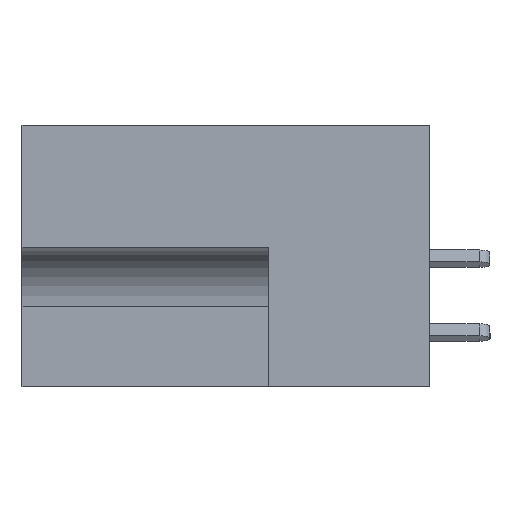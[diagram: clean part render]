
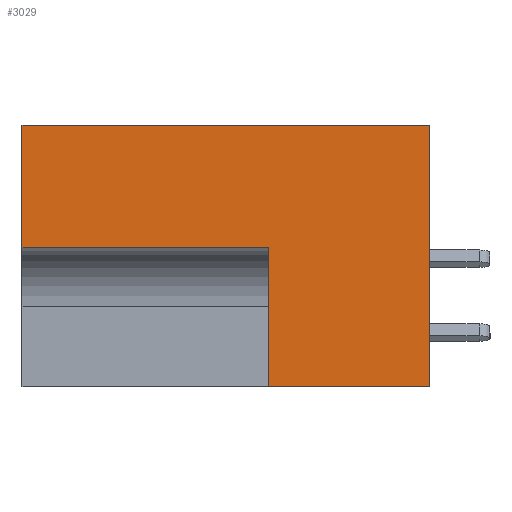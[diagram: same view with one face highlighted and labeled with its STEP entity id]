
A CAD part, left-side view. The second image highlights one B-rep face of the part: STEP entity #3029.
In plain terms, the highlighted planar face has unit normal (-1, 0, 0).
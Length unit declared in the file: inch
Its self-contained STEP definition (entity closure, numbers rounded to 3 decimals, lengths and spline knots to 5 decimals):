
#59 = EDGE_CURVE ( 'NONE', #28640, #12085, #19210, .T. ) ;
#116 = CARTESIAN_POINT ( 'NONE',  ( 0., 0.828, 0. ) ) ;
#3029 = ADVANCED_FACE ( 'NONE', ( #16331 ), #13114, .F. ) ;
#4414 = ORIENTED_EDGE ( 'NONE', *, *, #17054, .T. ) ;
#4541 = CARTESIAN_POINT ( 'NONE',  ( 0., 0.328, -0.248 ) ) ;
#5088 = CARTESIAN_POINT ( 'NONE',  ( 0., 0., -0.531 ) ) ;
#5208 = EDGE_CURVE ( 'NONE', #25098, #28640, #22709, .T. ) ;
#5227 = VECTOR ( 'NONE', #7574, 39.37008 ) ;
#5331 = VECTOR ( 'NONE', #13494, 39.37008 ) ;
#5976 = CARTESIAN_POINT ( 'NONE',  ( 0., 0.328, -0.248 ) ) ;
#7574 = DIRECTION ( 'NONE',  ( 0., 0., 1. ) ) ;
#8869 = EDGE_CURVE ( 'NONE', #22255, #29161, #20364, .T. ) ;
#9506 = LINE ( 'NONE', #26531, #28365 ) ;
#9760 = DIRECTION ( 'NONE',  ( 0., -1., 0. ) ) ;
#10424 = ORIENTED_EDGE ( 'NONE', *, *, #8869, .F. ) ;
#10444 = CARTESIAN_POINT ( 'NONE',  ( 0., 0.328, -0.531 ) ) ;
#12024 = CARTESIAN_POINT ( 'NONE',  ( 0., 0.453, 0. ) ) ;
#12085 = VERTEX_POINT ( 'NONE', #22172 ) ;
#12803 = CARTESIAN_POINT ( 'NONE',  ( 0., 0.453, 0. ) ) ;
#12969 = LINE ( 'NONE', #23345, #24132 ) ;
#13114 = PLANE ( 'NONE',  #18479 ) ;
#13494 = DIRECTION ( 'NONE',  ( 0., 1., 0. ) ) ;
#14579 = DIRECTION ( 'NONE',  ( 0., -1., 0. ) ) ;
#15883 = ORIENTED_EDGE ( 'NONE', *, *, #59, .F. ) ;
#16177 = VECTOR ( 'NONE', #27670, 39.37008 ) ;
#16331 = FACE_OUTER_BOUND ( 'NONE', #28832, .T. ) ;
#17054 = EDGE_CURVE ( 'NONE', #26045, #29161, #12969, .T. ) ;
#18417 = ORIENTED_EDGE ( 'NONE', *, *, #5208, .F. ) ;
#18479 = AXIS2_PLACEMENT_3D ( 'NONE', #12803, #27468, #22691 ) ;
#19210 = LINE ( 'NONE', #5976, #5331 ) ;
#20328 = CARTESIAN_POINT ( 'NONE',  ( 0., 0.828, 0. ) ) ;
#20364 = LINE ( 'NONE', #12024, #23021 ) ;
#21770 = LINE ( 'NONE', #116, #5227 ) ;
#22172 = CARTESIAN_POINT ( 'NONE',  ( 0., 0.828, -0.248 ) ) ;
#22255 = VERTEX_POINT ( 'NONE', #20328 ) ;
#22691 = DIRECTION ( 'NONE',  ( 0., 0., -1. ) ) ;
#22709 = LINE ( 'NONE', #10444, #16177 ) ;
#23021 = VECTOR ( 'NONE', #9760, 39.37008 ) ;
#23345 = CARTESIAN_POINT ( 'NONE',  ( 0., 0., 0. ) ) ;
#23838 = CARTESIAN_POINT ( 'NONE',  ( 0., 0., 0. ) ) ;
#24132 = VECTOR ( 'NONE', #27808, 39.37008 ) ;
#25098 = VERTEX_POINT ( 'NONE', #31263 ) ;
#26045 = VERTEX_POINT ( 'NONE', #5088 ) ;
#26531 = CARTESIAN_POINT ( 'NONE',  ( 0., 0.453, -0.531 ) ) ;
#27086 = EDGE_CURVE ( 'NONE', #25098, #26045, #9506, .T. ) ;
#27413 = EDGE_CURVE ( 'NONE', #12085, #22255, #21770, .T. ) ;
#27468 = DIRECTION ( 'NONE',  ( 1., 0., 0. ) ) ;
#27670 = DIRECTION ( 'NONE',  ( 0., 0., 1. ) ) ;
#27808 = DIRECTION ( 'NONE',  ( 0., 0., 1. ) ) ;
#28365 = VECTOR ( 'NONE', #14579, 39.37008 ) ;
#28640 = VERTEX_POINT ( 'NONE', #4541 ) ;
#28832 = EDGE_LOOP ( 'NONE', ( #30685, #15883, #18417, #30165, #4414, #10424 ) ) ;
#29161 = VERTEX_POINT ( 'NONE', #23838 ) ;
#30165 = ORIENTED_EDGE ( 'NONE', *, *, #27086, .T. ) ;
#30685 = ORIENTED_EDGE ( 'NONE', *, *, #27413, .F. ) ;
#31263 = CARTESIAN_POINT ( 'NONE',  ( 0., 0.328, -0.531 ) ) ;
